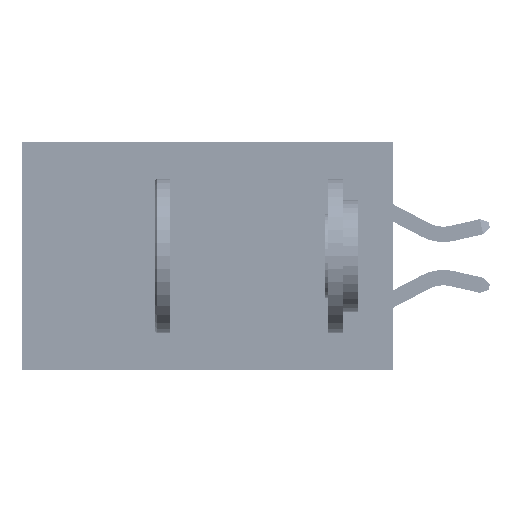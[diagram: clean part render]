
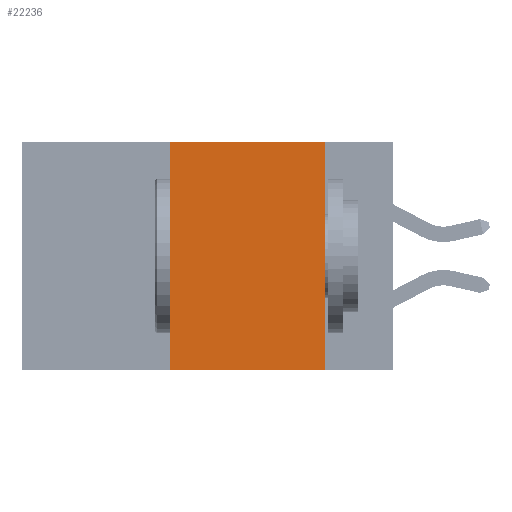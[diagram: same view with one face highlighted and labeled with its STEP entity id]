
A CAD part, left-side view. The second image highlights one B-rep face of the part: STEP entity #22236.
In plain terms, the highlighted planar face has unit normal (-1, 0, 0).
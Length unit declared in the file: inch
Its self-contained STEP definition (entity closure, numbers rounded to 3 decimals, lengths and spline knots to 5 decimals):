
#17 = LINE ( 'NONE', #10770, #11263 ) ;
#458 = PLANE ( 'NONE',  #30711 ) ;
#2910 = CARTESIAN_POINT ( 'NONE',  ( 0., 0.11, 0. ) ) ;
#3274 = CARTESIAN_POINT ( 'NONE',  ( 0., 0.36, -0.37 ) ) ;
#6910 = VERTEX_POINT ( 'NONE', #3274 ) ;
#10105 = ORIENTED_EDGE ( 'NONE', *, *, #44711, .T. ) ;
#10770 = CARTESIAN_POINT ( 'NONE',  ( 0., 0.6, -0.37 ) ) ;
#10804 = VERTEX_POINT ( 'NONE', #47408 ) ;
#10975 = CARTESIAN_POINT ( 'NONE',  ( 0., 0.6, 0. ) ) ;
#11002 = DIRECTION ( 'NONE',  ( 0., 0., 1. ) ) ;
#11263 = VECTOR ( 'NONE', #30404, 39.37008 ) ;
#12574 = VECTOR ( 'NONE', #48721, 39.37008 ) ;
#12797 = VERTEX_POINT ( 'NONE', #33105 ) ;
#14832 = DIRECTION ( 'NONE',  ( 0., -1., 0. ) ) ;
#14942 = EDGE_CURVE ( 'NONE', #10804, #44915, #18833, .T. ) ;
#16103 = ORIENTED_EDGE ( 'NONE', *, *, #43962, .F. ) ;
#17604 = VECTOR ( 'NONE', #14832, 39.37008 ) ;
#18833 = LINE ( 'NONE', #10975, #17604 ) ;
#22236 = ADVANCED_FACE ( 'NONE', ( #42488 ), #458, .F. ) ;
#24943 = CARTESIAN_POINT ( 'NONE',  ( 0., 0.11, 0. ) ) ;
#25752 = DIRECTION ( 'NONE',  ( 0., 0., -1. ) ) ;
#28135 = EDGE_LOOP ( 'NONE', ( #16103, #45633, #40821, #10105 ) ) ;
#29384 = LINE ( 'NONE', #24943, #12574 ) ;
#30404 = DIRECTION ( 'NONE',  ( 0., -1., 0. ) ) ;
#30711 = AXIS2_PLACEMENT_3D ( 'NONE', #31773, #48293, #25752 ) ;
#31773 = CARTESIAN_POINT ( 'NONE',  ( 0., 0.6, 0. ) ) ;
#33071 = VECTOR ( 'NONE', #11002, 39.37008 ) ;
#33105 = CARTESIAN_POINT ( 'NONE',  ( 0., 0.11, -0.37 ) ) ;
#37575 = EDGE_CURVE ( 'NONE', #6910, #10804, #41770, .T. ) ;
#40821 = ORIENTED_EDGE ( 'NONE', *, *, #37575, .F. ) ;
#41770 = LINE ( 'NONE', #43161, #33071 ) ;
#42488 = FACE_OUTER_BOUND ( 'NONE', #28135, .T. ) ;
#43161 = CARTESIAN_POINT ( 'NONE',  ( 0., 0.36, 0. ) ) ;
#43962 = EDGE_CURVE ( 'NONE', #44915, #12797, #29384, .T. ) ;
#44711 = EDGE_CURVE ( 'NONE', #6910, #12797, #17, .T. ) ;
#44915 = VERTEX_POINT ( 'NONE', #2910 ) ;
#45633 = ORIENTED_EDGE ( 'NONE', *, *, #14942, .F. ) ;
#47408 = CARTESIAN_POINT ( 'NONE',  ( 0., 0.36, 0. ) ) ;
#48293 = DIRECTION ( 'NONE',  ( 1., 0., 0. ) ) ;
#48721 = DIRECTION ( 'NONE',  ( 0., 0., -1. ) ) ;
